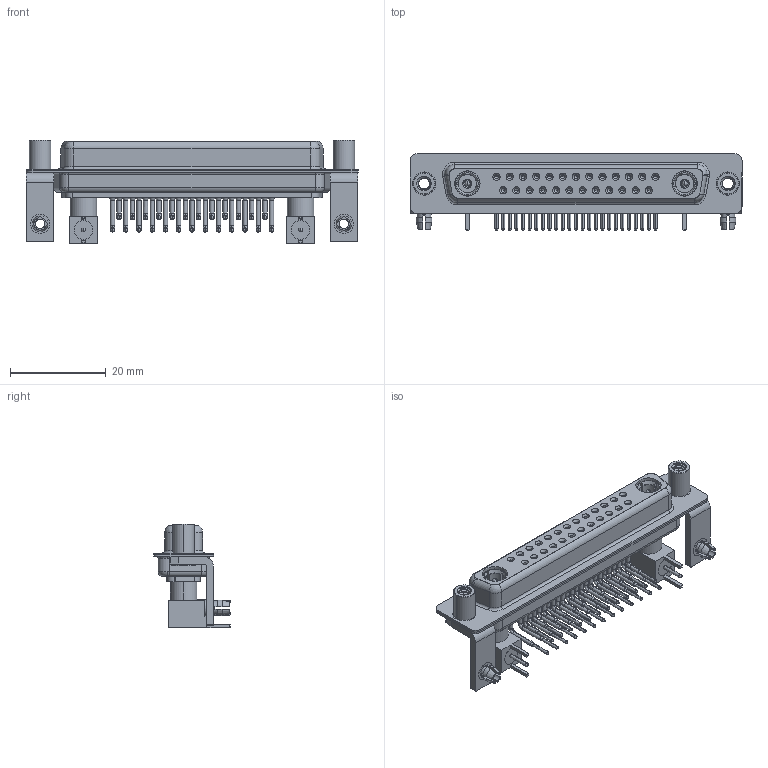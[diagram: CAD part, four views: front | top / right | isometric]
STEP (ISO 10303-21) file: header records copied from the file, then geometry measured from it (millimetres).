
FILE_DESCRIPTION (( 'STEP AP203' ), '1' );
FILE_NAME ('630-27W2240-7T5.STEP', '2022-06-07T13:36:18', ( '' ), ( '' ), 'SwSTEP 2.0', 'SolidWorks 2020', '' );
FILE_SCHEMA (( 'CONFIG_CONTROL_DESIGN' ));
Length unit declared in the file: millimetre
Products named in the file (17): 630Combo Shell Rear_37 Contacts; 630-27W2240-7T5; 630Combo Housing_27W2; 630Combo Contact Row 1; 630Combo Threaded Standoff_5; 630Combo Contact Row 2; Locking Collar; Co-Ax Plug_RA PC Tail; Co-Ax Plug Assy_RA; Pin_RA; 630Combo Stabilizer Bracket; RA Back Shell; Insulator RA Pin; 630Combo Board Lock; 630Combo Shell Front_37 Contacts; Insulator Pin_Straight PC Tail
Assembly tree (48 placements, depth 3):
  630-27W2240-7T5
    630Combo Housing_27W2
    630Combo Shell Front_37 Contacts
    630Combo Shell Rear_37 Contacts
    630Combo Stabilizer Bracket  x2
    630Combo Board Lock  x2
    630Combo Threaded Standoff_5  x2
    Co-Ax Plug Assy_RA
      Co-Ax Plug_RA PC Tail
      Insulator Pin_Straight PC Tail
      Pin_RA
      Locking Collar
      RA Back Shell
      Insulator RA Pin
    Co-Ax Plug Assy_RA
      Co-Ax Plug_RA PC Tail
      Insulator Pin_Straight PC Tail
      Pin_RA
      Locking Collar
      RA Back Shell
      Insulator RA Pin
    630Combo Contact Row 1  x13
    630Combo Contact Row 2  x12
Bounding box: 69.4 x 16 x 21.61 mm (x, y, z)
Volume: 6438.9 mm3; surface area: 14919.3 mm2
Topology: 46 solids, 46 shells, 2120 faces, 5346 edges, 3372 vertices
Faces by surface type: cylinder 934, plane 646, cone 355, bspline 108, torus 69, sphere 8
Entity records: 31637 total; most frequent: CARTESIAN_POINT 7012, DIRECTION 5007, ORIENTED_EDGE 4306, EDGE_CURVE 2153, AXIS2_PLACEMENT_3D 2058, VERTEX_POINT 1375, EDGE_LOOP 1104, CIRCLE 1103
